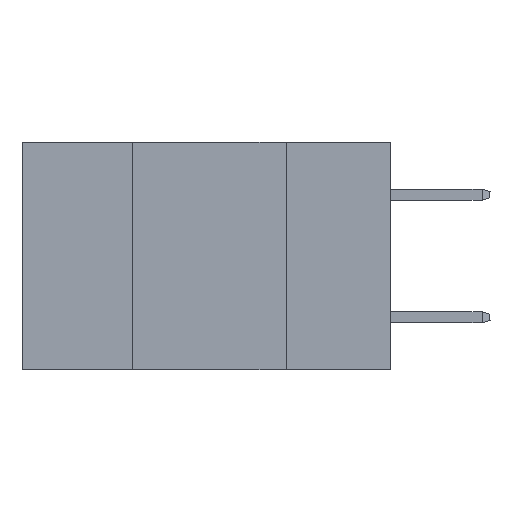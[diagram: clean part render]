
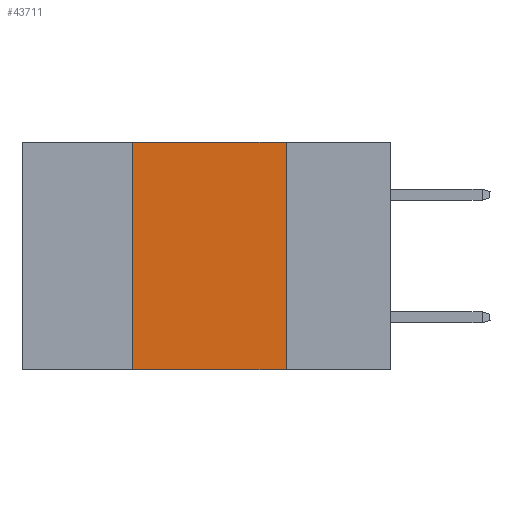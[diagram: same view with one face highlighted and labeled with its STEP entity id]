
A CAD part, left-side view. The second image highlights one B-rep face of the part: STEP entity #43711.
In plain terms, the highlighted planar face has unit normal (-1, 0, 0).
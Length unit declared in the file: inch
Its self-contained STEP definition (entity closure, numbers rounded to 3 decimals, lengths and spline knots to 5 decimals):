
#395 = CARTESIAN_POINT ( 'NONE',  ( 0., 0.42, 0. ) ) ;
#1372 = DIRECTION ( 'NONE',  ( 0., 0., 1. ) ) ;
#2492 = CARTESIAN_POINT ( 'NONE',  ( 0., 0.17, 0. ) ) ;
#5600 = CARTESIAN_POINT ( 'NONE',  ( 0., 0.6, 0. ) ) ;
#8755 = DIRECTION ( 'NONE',  ( 0., 0., -1. ) ) ;
#9011 = EDGE_CURVE ( 'NONE', #21200, #11022, #14083, .T. ) ;
#10945 = LINE ( 'NONE', #31369, #20697 ) ;
#11022 = VERTEX_POINT ( 'NONE', #2492 ) ;
#12142 = DIRECTION ( 'NONE',  ( 0., -1., 0. ) ) ;
#12363 = VERTEX_POINT ( 'NONE', #13678 ) ;
#12687 = VECTOR ( 'NONE', #12142, 39.37008 ) ;
#13678 = CARTESIAN_POINT ( 'NONE',  ( 0., 0.42, -0.37 ) ) ;
#14083 = LINE ( 'NONE', #35201, #31368 ) ;
#17035 = ORIENTED_EDGE ( 'NONE', *, *, #27226, .F. ) ;
#19667 = ORIENTED_EDGE ( 'NONE', *, *, #9011, .F. ) ;
#19921 = ORIENTED_EDGE ( 'NONE', *, *, #42457, .T. ) ;
#20697 = VECTOR ( 'NONE', #24165, 39.37008 ) ;
#21200 = VERTEX_POINT ( 'NONE', #395 ) ;
#21785 = FACE_OUTER_BOUND ( 'NONE', #42894, .T. ) ;
#22134 = CARTESIAN_POINT ( 'NONE',  ( 0., 0.6, -0.37 ) ) ;
#23931 = CARTESIAN_POINT ( 'NONE',  ( 0., 0.17, -0.37 ) ) ;
#24165 = DIRECTION ( 'NONE',  ( 0., 0., -1. ) ) ;
#25848 = PLANE ( 'NONE',  #41819 ) ;
#27226 = EDGE_CURVE ( 'NONE', #11022, #40706, #10945, .T. ) ;
#27597 = ORIENTED_EDGE ( 'NONE', *, *, #33933, .F. ) ;
#28977 = DIRECTION ( 'NONE',  ( 0., -1., 0. ) ) ;
#29281 = DIRECTION ( 'NONE',  ( 1., 0., 0. ) ) ;
#30515 = LINE ( 'NONE', #38819, #31616 ) ;
#31368 = VECTOR ( 'NONE', #28977, 39.37008 ) ;
#31369 = CARTESIAN_POINT ( 'NONE',  ( 0., 0.17, 0. ) ) ;
#31616 = VECTOR ( 'NONE', #1372, 39.37008 ) ;
#33933 = EDGE_CURVE ( 'NONE', #12363, #21200, #30515, .T. ) ;
#35201 = CARTESIAN_POINT ( 'NONE',  ( 0., 0.6, 0. ) ) ;
#38082 = LINE ( 'NONE', #22134, #12687 ) ;
#38819 = CARTESIAN_POINT ( 'NONE',  ( 0., 0.42, 0. ) ) ;
#40706 = VERTEX_POINT ( 'NONE', #23931 ) ;
#41819 = AXIS2_PLACEMENT_3D ( 'NONE', #5600, #29281, #8755 ) ;
#42457 = EDGE_CURVE ( 'NONE', #12363, #40706, #38082, .T. ) ;
#42894 = EDGE_LOOP ( 'NONE', ( #17035, #19667, #27597, #19921 ) ) ;
#43711 = ADVANCED_FACE ( 'NONE', ( #21785 ), #25848, .F. ) ;
